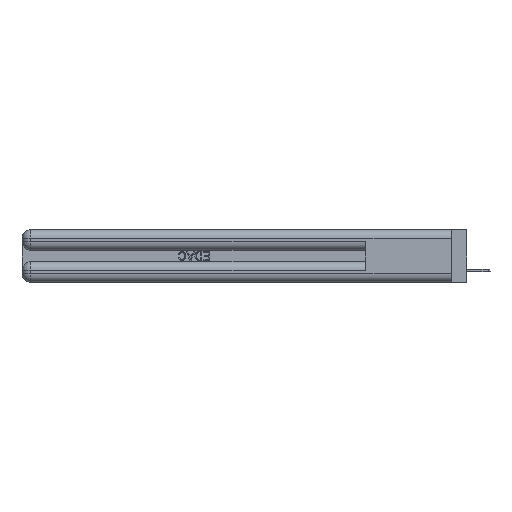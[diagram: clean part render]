
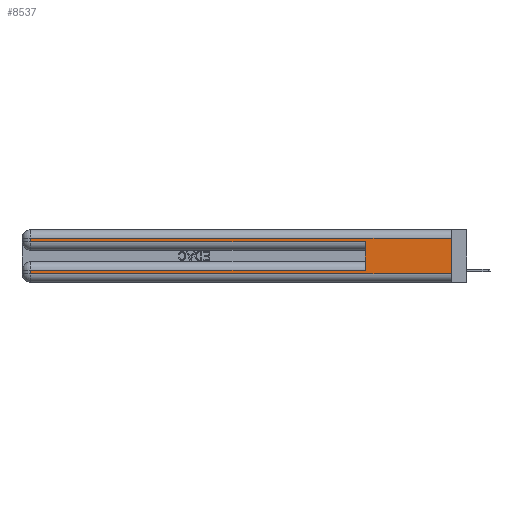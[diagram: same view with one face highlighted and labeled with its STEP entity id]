
A CAD part, left-side view. The second image highlights one B-rep face of the part: STEP entity #8537.
In plain terms, the highlighted planar face has unit normal (-1, 0, 0).
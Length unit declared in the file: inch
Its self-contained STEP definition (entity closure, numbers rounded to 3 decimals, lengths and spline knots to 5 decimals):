
#92 = CARTESIAN_POINT ( 'NONE',  ( 0., 0., 0.06 ) ) ;
#1855 = VERTEX_POINT ( 'NONE', #5813 ) ;
#2358 = CARTESIAN_POINT ( 'NONE',  ( 0., 2.94, 0.37 ) ) ;
#2419 = EDGE_CURVE ( 'NONE', #23121, #4696, #30794, .T. ) ;
#2560 = FACE_OUTER_BOUND ( 'NONE', #40074, .T. ) ;
#2802 = ORIENTED_EDGE ( 'NONE', *, *, #27048, .F. ) ;
#3534 = DIRECTION ( 'NONE',  ( 0., 0., -1. ) ) ;
#3704 = EDGE_CURVE ( 'NONE', #25036, #32720, #26240, .T. ) ;
#3962 = LINE ( 'NONE', #2358, #31457 ) ;
#4521 = DIRECTION ( 'NONE',  ( 0., 0., 1. ) ) ;
#4696 = VERTEX_POINT ( 'NONE', #38777 ) ;
#4824 = ORIENTED_EDGE ( 'NONE', *, *, #29672, .T. ) ;
#4939 = VECTOR ( 'NONE', #6287, 39.37008 ) ;
#5607 = VECTOR ( 'NONE', #14371, 39.37008 ) ;
#5675 = CARTESIAN_POINT ( 'NONE',  ( 0., 0., 0.37 ) ) ;
#5813 = CARTESIAN_POINT ( 'NONE',  ( 0., 2.94, 0.06 ) ) ;
#6287 = DIRECTION ( 'NONE',  ( 0., -1., 0. ) ) ;
#6830 = LINE ( 'NONE', #35246, #30936 ) ;
#7549 = CARTESIAN_POINT ( 'NONE',  ( 0., 0.6, 0.145 ) ) ;
#8537 = ADVANCED_FACE ( 'NONE', ( #2560 ), #27879, .F. ) ;
#9384 = ORIENTED_EDGE ( 'NONE', *, *, #3704, .T. ) ;
#9703 = DIRECTION ( 'NONE',  ( 0., -1., 0. ) ) ;
#10820 = LINE ( 'NONE', #31424, #4939 ) ;
#10985 = EDGE_CURVE ( 'NONE', #25036, #26511, #13630, .T. ) ;
#11171 = VECTOR ( 'NONE', #4521, 39.37008 ) ;
#13630 = LINE ( 'NONE', #7549, #11171 ) ;
#14371 = DIRECTION ( 'NONE',  ( 0., 1., 0. ) ) ;
#14811 = CARTESIAN_POINT ( 'NONE',  ( 0., 0., 0.06 ) ) ;
#14858 = DIRECTION ( 'NONE',  ( 0., 0., -1. ) ) ;
#18010 = CARTESIAN_POINT ( 'NONE',  ( 0., 0.6, 0.285 ) ) ;
#18562 = DIRECTION ( 'NONE',  ( 0., 0., -1. ) ) ;
#18692 = DIRECTION ( 'NONE',  ( 1., 0., 0. ) ) ;
#19503 = LINE ( 'NONE', #92, #21503 ) ;
#19956 = CARTESIAN_POINT ( 'NONE',  ( 0., 0., 0.31 ) ) ;
#20020 = ORIENTED_EDGE ( 'NONE', *, *, #25219, .T. ) ;
#20385 = DIRECTION ( 'NONE',  ( 0., 1., 0. ) ) ;
#21271 = CARTESIAN_POINT ( 'NONE',  ( 0., 0.6, 0.085 ) ) ;
#21503 = VECTOR ( 'NONE', #9703, 39.37008 ) ;
#23121 = VERTEX_POINT ( 'NONE', #24708 ) ;
#23581 = CARTESIAN_POINT ( 'NONE',  ( 0., 0., 0.37 ) ) ;
#23737 = EDGE_CURVE ( 'NONE', #4696, #33702, #6830, .T. ) ;
#24344 = ORIENTED_EDGE ( 'NONE', *, *, #10985, .F. ) ;
#24708 = CARTESIAN_POINT ( 'NONE',  ( 0., 0., 0.31 ) ) ;
#25036 = VERTEX_POINT ( 'NONE', #21271 ) ;
#25219 = EDGE_CURVE ( 'NONE', #1855, #30302, #19503, .T. ) ;
#25361 = ORIENTED_EDGE ( 'NONE', *, *, #29869, .T. ) ;
#25893 = CARTESIAN_POINT ( 'NONE',  ( 0., 2.94, 0.285 ) ) ;
#26235 = VECTOR ( 'NONE', #39106, 39.37008 ) ;
#26240 = LINE ( 'NONE', #30285, #5607 ) ;
#26511 = VERTEX_POINT ( 'NONE', #18010 ) ;
#26778 = ORIENTED_EDGE ( 'NONE', *, *, #23737, .T. ) ;
#27048 = EDGE_CURVE ( 'NONE', #23121, #30302, #34611, .T. ) ;
#27879 = PLANE ( 'NONE',  #30470 ) ;
#29672 = EDGE_CURVE ( 'NONE', #32720, #1855, #3962, .T. ) ;
#29720 = ORIENTED_EDGE ( 'NONE', *, *, #2419, .T. ) ;
#29784 = VECTOR ( 'NONE', #20385, 39.37008 ) ;
#29869 = EDGE_CURVE ( 'NONE', #33702, #26511, #10820, .T. ) ;
#30285 = CARTESIAN_POINT ( 'NONE',  ( 0., 0., 0.085 ) ) ;
#30302 = VERTEX_POINT ( 'NONE', #14811 ) ;
#30470 = AXIS2_PLACEMENT_3D ( 'NONE', #5675, #18692, #18562 ) ;
#30794 = LINE ( 'NONE', #19956, #29784 ) ;
#30936 = VECTOR ( 'NONE', #3534, 39.37008 ) ;
#31424 = CARTESIAN_POINT ( 'NONE',  ( 0., 0., 0.285 ) ) ;
#31457 = VECTOR ( 'NONE', #14858, 39.37008 ) ;
#32720 = VERTEX_POINT ( 'NONE', #38886 ) ;
#33702 = VERTEX_POINT ( 'NONE', #25893 ) ;
#34611 = LINE ( 'NONE', #23581, #26235 ) ;
#35246 = CARTESIAN_POINT ( 'NONE',  ( 0., 2.94, 0.37 ) ) ;
#38777 = CARTESIAN_POINT ( 'NONE',  ( 0., 2.94, 0.31 ) ) ;
#38886 = CARTESIAN_POINT ( 'NONE',  ( 0., 2.94, 0.085 ) ) ;
#39106 = DIRECTION ( 'NONE',  ( 0., 0., -1. ) ) ;
#40074 = EDGE_LOOP ( 'NONE', ( #2802, #29720, #26778, #25361, #24344, #9384, #4824, #20020 ) ) ;
